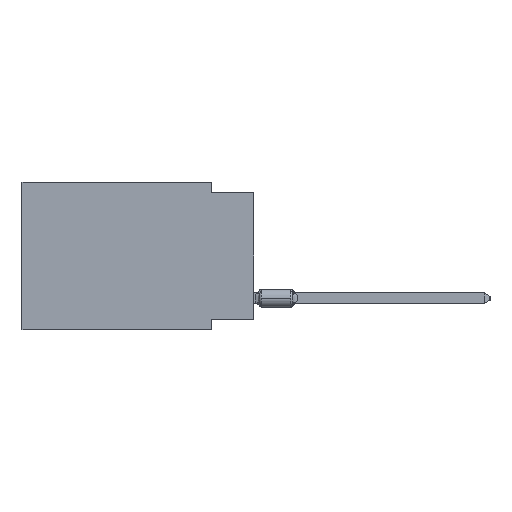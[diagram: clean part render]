
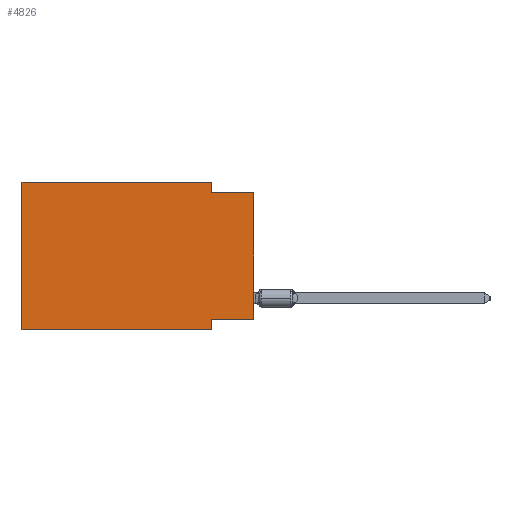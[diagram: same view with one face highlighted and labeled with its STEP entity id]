
A CAD part, left-side view. The second image highlights one B-rep face of the part: STEP entity #4826.
In plain terms, the highlighted planar face has unit normal (-1, 0, 0).
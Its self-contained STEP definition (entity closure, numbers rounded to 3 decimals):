
#572 = DIRECTION ( 'NONE',  ( 0., 0., -1. ) ) ;
#718 = VECTOR ( 'NONE', #39349, 1000. ) ;
#1606 = CARTESIAN_POINT ( 'NONE',  ( 0., 13.97, 0. ) ) ;
#3230 = CARTESIAN_POINT ( 'NONE',  ( 0., 0., -8.255 ) ) ;
#3326 = ORIENTED_EDGE ( 'NONE', *, *, #45030, .F. ) ;
#4035 = EDGE_LOOP ( 'NONE', ( #34680, #44238, #38774, #32887, #42253, #19936, #3326, #17014 ) ) ;
#4532 = CARTESIAN_POINT ( 'NONE',  ( 0., 2.54, -0.635 ) ) ;
#4826 = ADVANCED_FACE ( 'NONE', ( #41200 ), #9956, .F. ) ;
#4849 = VERTEX_POINT ( 'NONE', #7651 ) ;
#7651 = CARTESIAN_POINT ( 'NONE',  ( 0., 2.54, -8.89 ) ) ;
#7880 = AXIS2_PLACEMENT_3D ( 'NONE', #23844, #37765, #572 ) ;
#8804 = LINE ( 'NONE', #15165, #718 ) ;
#9505 = VERTEX_POINT ( 'NONE', #38263 ) ;
#9956 = PLANE ( 'NONE',  #7880 ) ;
#10157 = DIRECTION ( 'NONE',  ( 0., 0., 1. ) ) ;
#10386 = LINE ( 'NONE', #30920, #31198 ) ;
#11308 = EDGE_CURVE ( 'NONE', #9505, #43290, #8804, .T. ) ;
#12518 = CARTESIAN_POINT ( 'NONE',  ( 0., 2.54, -8.89 ) ) ;
#12782 = LINE ( 'NONE', #1606, #38775 ) ;
#13577 = CARTESIAN_POINT ( 'NONE',  ( 0., 0., -0.635 ) ) ;
#15092 = EDGE_CURVE ( 'NONE', #44942, #19355, #17469, .T. ) ;
#15165 = CARTESIAN_POINT ( 'NONE',  ( 0., 13.97, 0. ) ) ;
#15690 = DIRECTION ( 'NONE',  ( 0., 0., -1. ) ) ;
#15752 = EDGE_CURVE ( 'NONE', #32378, #19355, #10386, .T. ) ;
#16795 = EDGE_CURVE ( 'NONE', #34239, #44942, #25696, .T. ) ;
#17014 = ORIENTED_EDGE ( 'NONE', *, *, #34575, .F. ) ;
#17025 = CARTESIAN_POINT ( 'NONE',  ( 0., 13.97, -8.89 ) ) ;
#17311 = VECTOR ( 'NONE', #39615, 1000. ) ;
#17469 = LINE ( 'NONE', #38922, #28242 ) ;
#18844 = CARTESIAN_POINT ( 'NONE',  ( 0., 2.54, 0. ) ) ;
#19355 = VERTEX_POINT ( 'NONE', #13577 ) ;
#19936 = ORIENTED_EDGE ( 'NONE', *, *, #25504, .T. ) ;
#20874 = DIRECTION ( 'NONE',  ( 0., -1., 0. ) ) ;
#23810 = EDGE_CURVE ( 'NONE', #43290, #34239, #12782, .T. ) ;
#23844 = CARTESIAN_POINT ( 'NONE',  ( 0., 13.97, 0. ) ) ;
#25504 = EDGE_CURVE ( 'NONE', #9505, #4849, #33927, .T. ) ;
#25609 = VERTEX_POINT ( 'NONE', #34592 ) ;
#25696 = LINE ( 'NONE', #18844, #17311 ) ;
#27294 = DIRECTION ( 'NONE',  ( 0., -1., 0. ) ) ;
#28242 = VECTOR ( 'NONE', #20874, 1000. ) ;
#30154 = DIRECTION ( 'NONE',  ( 0., 1., 0. ) ) ;
#30374 = VECTOR ( 'NONE', #15690, 1000. ) ;
#30920 = CARTESIAN_POINT ( 'NONE',  ( 0., 0., 0. ) ) ;
#31028 = LINE ( 'NONE', #3230, #31838 ) ;
#31198 = VECTOR ( 'NONE', #10157, 1000. ) ;
#31838 = VECTOR ( 'NONE', #30154, 1000. ) ;
#32378 = VERTEX_POINT ( 'NONE', #33037 ) ;
#32887 = ORIENTED_EDGE ( 'NONE', *, *, #23810, .F. ) ;
#33037 = CARTESIAN_POINT ( 'NONE',  ( 0., 0., -8.255 ) ) ;
#33832 = CARTESIAN_POINT ( 'NONE',  ( 0., 13.97, 0. ) ) ;
#33927 = LINE ( 'NONE', #17025, #37356 ) ;
#34239 = VERTEX_POINT ( 'NONE', #35007 ) ;
#34575 = EDGE_CURVE ( 'NONE', #32378, #25609, #31028, .T. ) ;
#34592 = CARTESIAN_POINT ( 'NONE',  ( 0., 2.54, -8.255 ) ) ;
#34680 = ORIENTED_EDGE ( 'NONE', *, *, #15752, .T. ) ;
#35007 = CARTESIAN_POINT ( 'NONE',  ( 0., 2.54, 0. ) ) ;
#37356 = VECTOR ( 'NONE', #27294, 1000. ) ;
#37765 = DIRECTION ( 'NONE',  ( 1., 0., 0. ) ) ;
#38263 = CARTESIAN_POINT ( 'NONE',  ( 0., 13.97, -8.89 ) ) ;
#38774 = ORIENTED_EDGE ( 'NONE', *, *, #16795, .F. ) ;
#38775 = VECTOR ( 'NONE', #43331, 1000. ) ;
#38922 = CARTESIAN_POINT ( 'NONE',  ( 0., 0., -0.635 ) ) ;
#39349 = DIRECTION ( 'NONE',  ( 0., 0., 1. ) ) ;
#39615 = DIRECTION ( 'NONE',  ( 0., 0., -1. ) ) ;
#40348 = LINE ( 'NONE', #12518, #30374 ) ;
#41200 = FACE_OUTER_BOUND ( 'NONE', #4035, .T. ) ;
#42253 = ORIENTED_EDGE ( 'NONE', *, *, #11308, .F. ) ;
#43290 = VERTEX_POINT ( 'NONE', #33832 ) ;
#43331 = DIRECTION ( 'NONE',  ( 0., -1., 0. ) ) ;
#44238 = ORIENTED_EDGE ( 'NONE', *, *, #15092, .F. ) ;
#44942 = VERTEX_POINT ( 'NONE', #4532 ) ;
#45030 = EDGE_CURVE ( 'NONE', #25609, #4849, #40348, .T. ) ;
